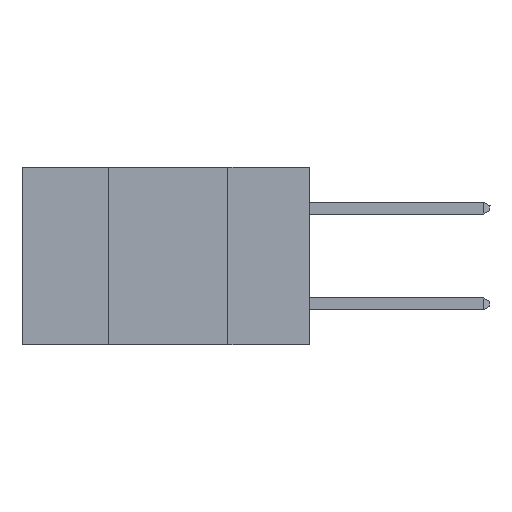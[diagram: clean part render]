
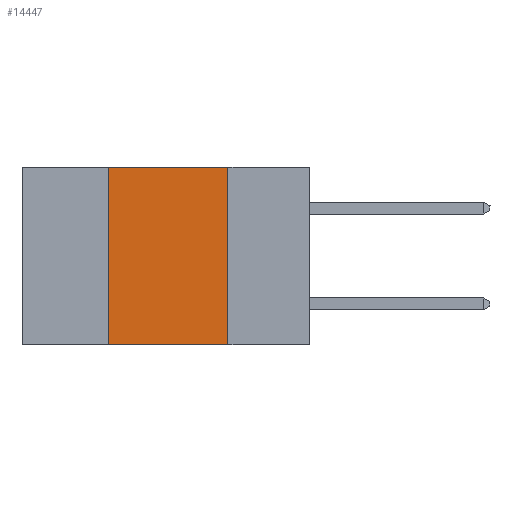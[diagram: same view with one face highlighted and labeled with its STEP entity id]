
A CAD part, left-side view. The second image highlights one B-rep face of the part: STEP entity #14447.
In plain terms, the highlighted planar face has unit normal (-1, 0, 0).
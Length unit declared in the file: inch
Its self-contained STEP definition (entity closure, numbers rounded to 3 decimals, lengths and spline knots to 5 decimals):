
#461 = DIRECTION ( 'NONE',  ( 1., 0., 0. ) ) ;
#636 = LINE ( 'NONE', #5159, #12499 ) ;
#871 = DIRECTION ( 'NONE',  ( 0., 0., 1. ) ) ;
#932 = ORIENTED_EDGE ( 'NONE', *, *, #6470, .F. ) ;
#2123 = CARTESIAN_POINT ( 'NONE',  ( 0., 0.6, -0.37 ) ) ;
#2199 = ORIENTED_EDGE ( 'NONE', *, *, #14512, .F. ) ;
#2241 = EDGE_CURVE ( 'NONE', #6103, #8121, #3724, .T. ) ;
#2656 = EDGE_CURVE ( 'NONE', #6103, #7016, #3873, .T. ) ;
#3724 = LINE ( 'NONE', #5374, #8920 ) ;
#3873 = LINE ( 'NONE', #2123, #6740 ) ;
#4374 = AXIS2_PLACEMENT_3D ( 'NONE', #9512, #461, #13072 ) ;
#4820 = CARTESIAN_POINT ( 'NONE',  ( 0., 0.42, -0.37 ) ) ;
#5159 = CARTESIAN_POINT ( 'NONE',  ( 0., 0.17, 0. ) ) ;
#5374 = CARTESIAN_POINT ( 'NONE',  ( 0., 0.42, 0. ) ) ;
#6103 = VERTEX_POINT ( 'NONE', #4820 ) ;
#6470 = EDGE_CURVE ( 'NONE', #8121, #9970, #12402, .T. ) ;
#6726 = DIRECTION ( 'NONE',  ( 0., -1., 0. ) ) ;
#6740 = VECTOR ( 'NONE', #6726, 39.37008 ) ;
#7016 = VERTEX_POINT ( 'NONE', #8216 ) ;
#8121 = VERTEX_POINT ( 'NONE', #11229 ) ;
#8216 = CARTESIAN_POINT ( 'NONE',  ( 0., 0.17, -0.37 ) ) ;
#8920 = VECTOR ( 'NONE', #871, 39.37008 ) ;
#9308 = VECTOR ( 'NONE', #13706, 39.37008 ) ;
#9512 = CARTESIAN_POINT ( 'NONE',  ( 0., 0.6, 0. ) ) ;
#9854 = ORIENTED_EDGE ( 'NONE', *, *, #2241, .F. ) ;
#9970 = VERTEX_POINT ( 'NONE', #11233 ) ;
#10494 = FACE_OUTER_BOUND ( 'NONE', #11661, .T. ) ;
#11229 = CARTESIAN_POINT ( 'NONE',  ( 0., 0.42, 0. ) ) ;
#11233 = CARTESIAN_POINT ( 'NONE',  ( 0., 0.17, 0. ) ) ;
#11661 = EDGE_LOOP ( 'NONE', ( #2199, #932, #9854, #12485 ) ) ;
#11760 = PLANE ( 'NONE',  #4374 ) ;
#12402 = LINE ( 'NONE', #13557, #9308 ) ;
#12485 = ORIENTED_EDGE ( 'NONE', *, *, #2656, .T. ) ;
#12499 = VECTOR ( 'NONE', #13233, 39.37008 ) ;
#13072 = DIRECTION ( 'NONE',  ( 0., 0., -1. ) ) ;
#13233 = DIRECTION ( 'NONE',  ( 0., 0., -1. ) ) ;
#13557 = CARTESIAN_POINT ( 'NONE',  ( 0., 0.6, 0. ) ) ;
#13706 = DIRECTION ( 'NONE',  ( 0., -1., 0. ) ) ;
#14447 = ADVANCED_FACE ( 'NONE', ( #10494 ), #11760, .F. ) ;
#14512 = EDGE_CURVE ( 'NONE', #9970, #7016, #636, .T. ) ;
